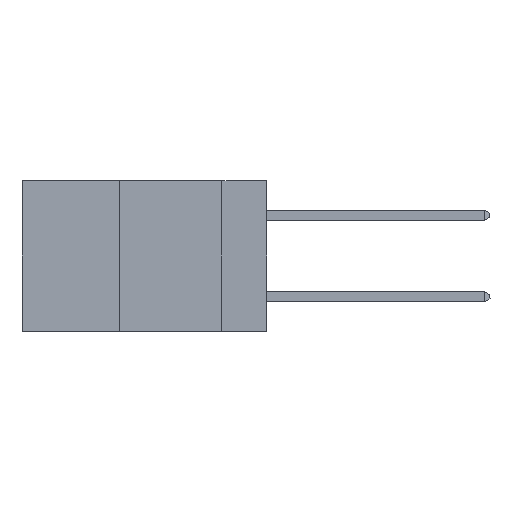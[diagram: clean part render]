
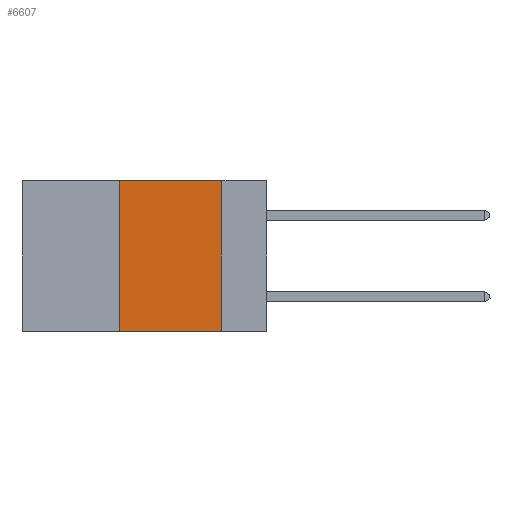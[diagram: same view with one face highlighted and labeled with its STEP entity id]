
A CAD part, left-side view. The second image highlights one B-rep face of the part: STEP entity #6607.
In plain terms, the highlighted planar face has unit normal (-1, 0, 0).
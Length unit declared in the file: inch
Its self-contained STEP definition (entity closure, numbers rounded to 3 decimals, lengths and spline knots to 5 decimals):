
#264 = VECTOR ( 'NONE', #10818, 39.37008 ) ;
#521 = AXIS2_PLACEMENT_3D ( 'NONE', #15635, #4506, #17523 ) ;
#609 = VECTOR ( 'NONE', #4682, 39.37008 ) ;
#2625 = PLANE ( 'NONE',  #521 ) ;
#3054 = DIRECTION ( 'NONE',  ( 0., -1., 0. ) ) ;
#3140 = VECTOR ( 'NONE', #6412, 39.37008 ) ;
#3645 = ORIENTED_EDGE ( 'NONE', *, *, #6101, .F. ) ;
#3758 = VERTEX_POINT ( 'NONE', #15105 ) ;
#4506 = DIRECTION ( 'NONE',  ( 1., 0., 0. ) ) ;
#4658 = VECTOR ( 'NONE', #3054, 39.37008 ) ;
#4682 = DIRECTION ( 'NONE',  ( 0., -1., 0. ) ) ;
#4705 = EDGE_CURVE ( 'NONE', #3758, #16875, #9759, .T. ) ;
#5660 = LINE ( 'NONE', #6537, #609 ) ;
#6101 = EDGE_CURVE ( 'NONE', #16875, #16816, #9118, .T. ) ;
#6412 = DIRECTION ( 'NONE',  ( 0., 0., -1. ) ) ;
#6537 = CARTESIAN_POINT ( 'NONE',  ( 0., 0.6, -0.37 ) ) ;
#6607 = ADVANCED_FACE ( 'NONE', ( #10222 ), #2625, .F. ) ;
#7248 = CARTESIAN_POINT ( 'NONE',  ( 0., 0.36, 0. ) ) ;
#7299 = EDGE_CURVE ( 'NONE', #16816, #18096, #22059, .T. ) ;
#7893 = ORIENTED_EDGE ( 'NONE', *, *, #7299, .F. ) ;
#9118 = LINE ( 'NONE', #14277, #4658 ) ;
#9250 = CARTESIAN_POINT ( 'NONE',  ( 0., 0.11, 0. ) ) ;
#9759 = LINE ( 'NONE', #21650, #264 ) ;
#10222 = FACE_OUTER_BOUND ( 'NONE', #12897, .T. ) ;
#10818 = DIRECTION ( 'NONE',  ( 0., 0., 1. ) ) ;
#12897 = EDGE_LOOP ( 'NONE', ( #7893, #3645, #17430, #16490 ) ) ;
#14277 = CARTESIAN_POINT ( 'NONE',  ( 0., 0.6, 0. ) ) ;
#15105 = CARTESIAN_POINT ( 'NONE',  ( 0., 0.36, -0.37 ) ) ;
#15213 = EDGE_CURVE ( 'NONE', #3758, #18096, #5660, .T. ) ;
#15635 = CARTESIAN_POINT ( 'NONE',  ( 0., 0.6, 0. ) ) ;
#16490 = ORIENTED_EDGE ( 'NONE', *, *, #15213, .T. ) ;
#16816 = VERTEX_POINT ( 'NONE', #9250 ) ;
#16875 = VERTEX_POINT ( 'NONE', #7248 ) ;
#17430 = ORIENTED_EDGE ( 'NONE', *, *, #4705, .F. ) ;
#17494 = CARTESIAN_POINT ( 'NONE',  ( 0., 0.11, 0. ) ) ;
#17523 = DIRECTION ( 'NONE',  ( 0., 0., -1. ) ) ;
#18096 = VERTEX_POINT ( 'NONE', #20211 ) ;
#20211 = CARTESIAN_POINT ( 'NONE',  ( 0., 0.11, -0.37 ) ) ;
#21650 = CARTESIAN_POINT ( 'NONE',  ( 0., 0.36, 0. ) ) ;
#22059 = LINE ( 'NONE', #17494, #3140 ) ;
